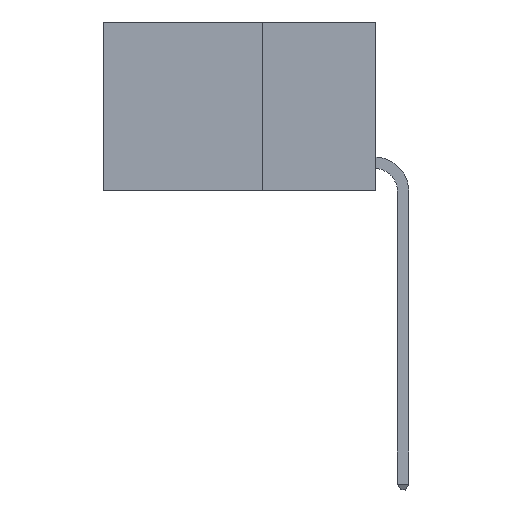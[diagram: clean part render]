
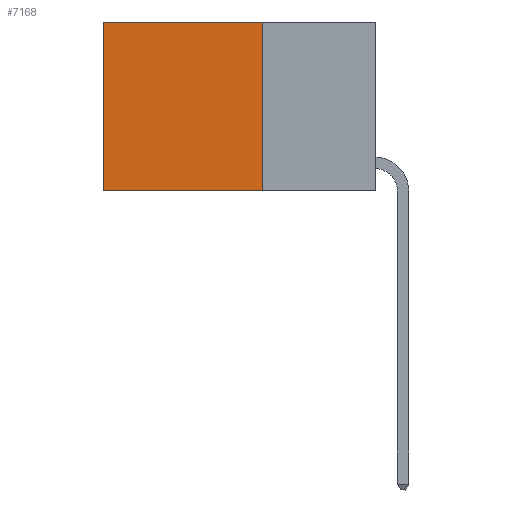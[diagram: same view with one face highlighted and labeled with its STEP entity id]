
A CAD part, left-side view. The second image highlights one B-rep face of the part: STEP entity #7168.
In plain terms, the highlighted planar face has unit normal (-1, 0, 0).
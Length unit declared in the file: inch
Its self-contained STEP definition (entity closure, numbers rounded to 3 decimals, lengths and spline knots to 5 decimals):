
#186 = FACE_OUTER_BOUND ( 'NONE', #8543, .T. ) ;
#374 = CARTESIAN_POINT ( 'NONE',  ( 0.2625, 0.6, -0.37 ) ) ;
#761 = CARTESIAN_POINT ( 'NONE',  ( 0.2625, 0.25, 0. ) ) ;
#1070 = DIRECTION ( 'NONE',  ( 0., 0., -1. ) ) ;
#1115 = DIRECTION ( 'NONE',  ( 0., 1., 0. ) ) ;
#1269 = LINE ( 'NONE', #17583, #7284 ) ;
#2378 = VECTOR ( 'NONE', #1070, 39.37008 ) ;
#2425 = CARTESIAN_POINT ( 'NONE',  ( 0.2625, 0.25, 0. ) ) ;
#2523 = CARTESIAN_POINT ( 'NONE',  ( 0.2625, 0.25, -0.37 ) ) ;
#2670 = EDGE_CURVE ( 'NONE', #15605, #3026, #10401, .T. ) ;
#3026 = VERTEX_POINT ( 'NONE', #374 ) ;
#3991 = CARTESIAN_POINT ( 'NONE',  ( 0.2625, 0.6, 0. ) ) ;
#4187 = CARTESIAN_POINT ( 'NONE',  ( 0.2625, 0.25, -0.37 ) ) ;
#6335 = CARTESIAN_POINT ( 'NONE',  ( 0.2625, 0.25, 0. ) ) ;
#7168 = ADVANCED_FACE ( 'NONE', ( #186 ), #16162, .F. ) ;
#7284 = VECTOR ( 'NONE', #7905, 39.37008 ) ;
#7813 = EDGE_CURVE ( 'NONE', #13738, #3026, #1269, .T. ) ;
#7855 = CARTESIAN_POINT ( 'NONE',  ( 0.2625, 0.25, 0. ) ) ;
#7905 = DIRECTION ( 'NONE',  ( 0., 0., -1. ) ) ;
#8543 = EDGE_LOOP ( 'NONE', ( #13545, #14639, #10056, #14490 ) ) ;
#9244 = DIRECTION ( 'NONE',  ( 0., 0., -1. ) ) ;
#10056 = ORIENTED_EDGE ( 'NONE', *, *, #11775, .F. ) ;
#10401 = LINE ( 'NONE', #2523, #17330 ) ;
#11775 = EDGE_CURVE ( 'NONE', #15353, #15605, #13834, .T. ) ;
#13467 = AXIS2_PLACEMENT_3D ( 'NONE', #7855, #17549, #9244 ) ;
#13545 = ORIENTED_EDGE ( 'NONE', *, *, #7813, .T. ) ;
#13738 = VERTEX_POINT ( 'NONE', #3991 ) ;
#13834 = LINE ( 'NONE', #2425, #2378 ) ;
#14490 = ORIENTED_EDGE ( 'NONE', *, *, #14640, .T. ) ;
#14614 = DIRECTION ( 'NONE',  ( 0., 1., 0. ) ) ;
#14639 = ORIENTED_EDGE ( 'NONE', *, *, #2670, .F. ) ;
#14640 = EDGE_CURVE ( 'NONE', #15353, #13738, #15855, .T. ) ;
#15003 = VECTOR ( 'NONE', #14614, 39.37008 ) ;
#15353 = VERTEX_POINT ( 'NONE', #6335 ) ;
#15605 = VERTEX_POINT ( 'NONE', #4187 ) ;
#15855 = LINE ( 'NONE', #761, #15003 ) ;
#16162 = PLANE ( 'NONE',  #13467 ) ;
#17330 = VECTOR ( 'NONE', #1115, 39.37008 ) ;
#17549 = DIRECTION ( 'NONE',  ( 1., 0., 0. ) ) ;
#17583 = CARTESIAN_POINT ( 'NONE',  ( 0.2625, 0.6, 0. ) ) ;
